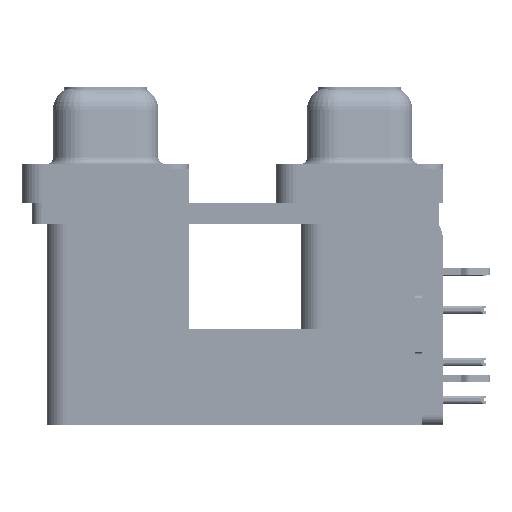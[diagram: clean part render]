
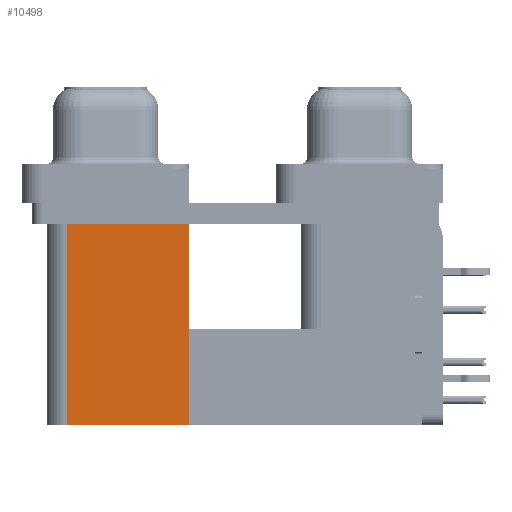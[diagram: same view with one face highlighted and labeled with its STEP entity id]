
A CAD part, left-side view. The second image highlights one B-rep face of the part: STEP entity #10498.
In plain terms, the highlighted planar face has unit normal (-1, 0, 0).
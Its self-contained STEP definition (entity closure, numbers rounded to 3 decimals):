
#3195 = DIRECTION ( 'NONE',  ( 1., 0., 0. ) ) ;
#3974 = EDGE_CURVE ( 'NONE', #69602, #20420, #45419, .T. ) ;
#9717 = CARTESIAN_POINT ( 'NONE',  ( 3.79, 12.775, -2.5 ) ) ;
#10498 = ADVANCED_FACE ( 'NONE', ( #71907 ), #66247, .F. ) ;
#10855 = EDGE_LOOP ( 'NONE', ( #56448, #62266, #52288, #24262 ) ) ;
#12826 = CARTESIAN_POINT ( 'NONE',  ( 3.79, 12.775, -2.5 ) ) ;
#12905 = CARTESIAN_POINT ( 'NONE',  ( 3.79, 21.975, -19.2 ) ) ;
#14212 = CARTESIAN_POINT ( 'NONE',  ( 3.79, 12.775, -19.2 ) ) ;
#17668 = DIRECTION ( 'NONE',  ( 0., 0., 1. ) ) ;
#20420 = VERTEX_POINT ( 'NONE', #57574 ) ;
#21068 = VECTOR ( 'NONE', #26568, 1000. ) ;
#24262 = ORIENTED_EDGE ( 'NONE', *, *, #45950, .T. ) ;
#26568 = DIRECTION ( 'NONE',  ( 0., 0., 1. ) ) ;
#26678 = LINE ( 'NONE', #9717, #28948 ) ;
#28003 = EDGE_CURVE ( 'NONE', #38782, #20420, #26678, .T. ) ;
#28948 = VECTOR ( 'NONE', #73868, 1000. ) ;
#28970 = LINE ( 'NONE', #69383, #71683 ) ;
#34802 = CARTESIAN_POINT ( 'NONE',  ( 3.79, 12.775, -19.2 ) ) ;
#38782 = VERTEX_POINT ( 'NONE', #12826 ) ;
#45419 = LINE ( 'NONE', #62068, #21068 ) ;
#45504 = EDGE_CURVE ( 'NONE', #68931, #69602, #51841, .T. ) ;
#45950 = EDGE_CURVE ( 'NONE', #68931, #38782, #28970, .T. ) ;
#47372 = DIRECTION ( 'NONE',  ( 0., 0., -1. ) ) ;
#51146 = VECTOR ( 'NONE', #69193, 1000. ) ;
#51841 = LINE ( 'NONE', #34802, #51146 ) ;
#52288 = ORIENTED_EDGE ( 'NONE', *, *, #45504, .F. ) ;
#56448 = ORIENTED_EDGE ( 'NONE', *, *, #28003, .T. ) ;
#57574 = CARTESIAN_POINT ( 'NONE',  ( 3.79, 21.975, -2.5 ) ) ;
#60590 = CARTESIAN_POINT ( 'NONE',  ( 3.79, 12.775, -19.2 ) ) ;
#62068 = CARTESIAN_POINT ( 'NONE',  ( 3.79, 21.975, -19.2 ) ) ;
#62266 = ORIENTED_EDGE ( 'NONE', *, *, #3974, .F. ) ;
#66247 = PLANE ( 'NONE',  #71707 ) ;
#68931 = VERTEX_POINT ( 'NONE', #14212 ) ;
#69193 = DIRECTION ( 'NONE',  ( 0., 1., 0. ) ) ;
#69383 = CARTESIAN_POINT ( 'NONE',  ( 3.79, 12.775, -19.2 ) ) ;
#69602 = VERTEX_POINT ( 'NONE', #12905 ) ;
#71683 = VECTOR ( 'NONE', #17668, 1000. ) ;
#71707 = AXIS2_PLACEMENT_3D ( 'NONE', #60590, #3195, #47372 ) ;
#71907 = FACE_OUTER_BOUND ( 'NONE', #10855, .T. ) ;
#73868 = DIRECTION ( 'NONE',  ( 0., 1., 0. ) ) ;
